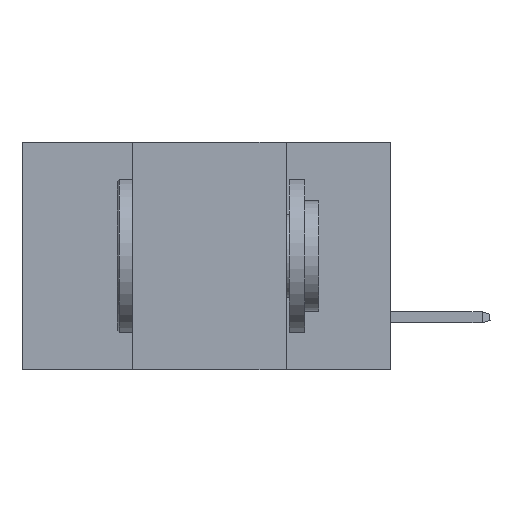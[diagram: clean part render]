
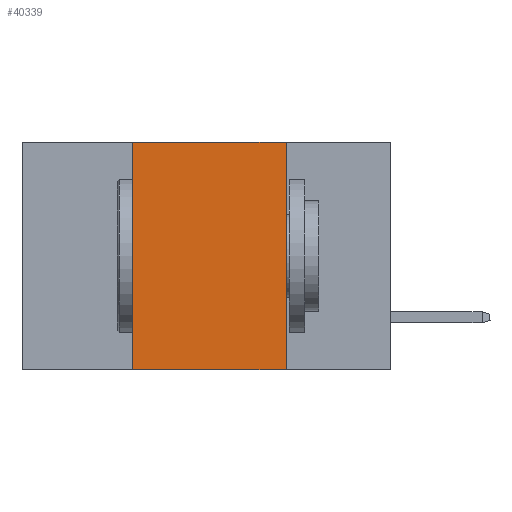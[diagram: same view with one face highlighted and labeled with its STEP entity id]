
A CAD part, left-side view. The second image highlights one B-rep face of the part: STEP entity #40339.
In plain terms, the highlighted planar face has unit normal (-1, 0, 0).
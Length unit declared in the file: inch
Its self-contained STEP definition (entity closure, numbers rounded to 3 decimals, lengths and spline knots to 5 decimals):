
#137 = EDGE_CURVE ( 'NONE', #1799, #35595, #14537, .T. ) ;
#934 = CARTESIAN_POINT ( 'NONE',  ( 0., 0.6, -0.37 ) ) ;
#1240 = CARTESIAN_POINT ( 'NONE',  ( 0., 0.6, 0. ) ) ;
#1799 = VERTEX_POINT ( 'NONE', #46454 ) ;
#2294 = EDGE_CURVE ( 'NONE', #8591, #1799, #25864, .T. ) ;
#3085 = AXIS2_PLACEMENT_3D ( 'NONE', #1240, #35552, #27461 ) ;
#5699 = VECTOR ( 'NONE', #27046, 39.37008 ) ;
#5988 = CARTESIAN_POINT ( 'NONE',  ( 0., 0.42, -0.37 ) ) ;
#6865 = ORIENTED_EDGE ( 'NONE', *, *, #15704, .T. ) ;
#7298 = VECTOR ( 'NONE', #44834, 39.37008 ) ;
#8591 = VERTEX_POINT ( 'NONE', #9974 ) ;
#8801 = ORIENTED_EDGE ( 'NONE', *, *, #137, .F. ) ;
#9690 = LINE ( 'NONE', #32871, #7298 ) ;
#9974 = CARTESIAN_POINT ( 'NONE',  ( 0., 0.42, 0. ) ) ;
#10032 = VERTEX_POINT ( 'NONE', #5988 ) ;
#11274 = EDGE_LOOP ( 'NONE', ( #8801, #44836, #16982, #6865 ) ) ;
#12844 = EDGE_CURVE ( 'NONE', #10032, #8591, #9690, .T. ) ;
#14537 = LINE ( 'NONE', #35900, #18660 ) ;
#15704 = EDGE_CURVE ( 'NONE', #10032, #35595, #16400, .T. ) ;
#16400 = LINE ( 'NONE', #934, #49153 ) ;
#16982 = ORIENTED_EDGE ( 'NONE', *, *, #12844, .F. ) ;
#17691 = CARTESIAN_POINT ( 'NONE',  ( 0., 0.17, -0.37 ) ) ;
#18660 = VECTOR ( 'NONE', #23937, 39.37008 ) ;
#23010 = CARTESIAN_POINT ( 'NONE',  ( 0., 0.6, 0. ) ) ;
#23937 = DIRECTION ( 'NONE',  ( 0., 0., -1. ) ) ;
#25864 = LINE ( 'NONE', #23010, #5699 ) ;
#27046 = DIRECTION ( 'NONE',  ( 0., -1., 0. ) ) ;
#27461 = DIRECTION ( 'NONE',  ( 0., 0., -1. ) ) ;
#31101 = PLANE ( 'NONE',  #3085 ) ;
#32871 = CARTESIAN_POINT ( 'NONE',  ( 0., 0.42, 0. ) ) ;
#35259 = DIRECTION ( 'NONE',  ( 0., -1., 0. ) ) ;
#35552 = DIRECTION ( 'NONE',  ( 1., 0., 0. ) ) ;
#35595 = VERTEX_POINT ( 'NONE', #17691 ) ;
#35900 = CARTESIAN_POINT ( 'NONE',  ( 0., 0.17, 0. ) ) ;
#40339 = ADVANCED_FACE ( 'NONE', ( #48728 ), #31101, .F. ) ;
#44834 = DIRECTION ( 'NONE',  ( 0., 0., 1. ) ) ;
#44836 = ORIENTED_EDGE ( 'NONE', *, *, #2294, .F. ) ;
#46454 = CARTESIAN_POINT ( 'NONE',  ( 0., 0.17, 0. ) ) ;
#48728 = FACE_OUTER_BOUND ( 'NONE', #11274, .T. ) ;
#49153 = VECTOR ( 'NONE', #35259, 39.37008 ) ;
